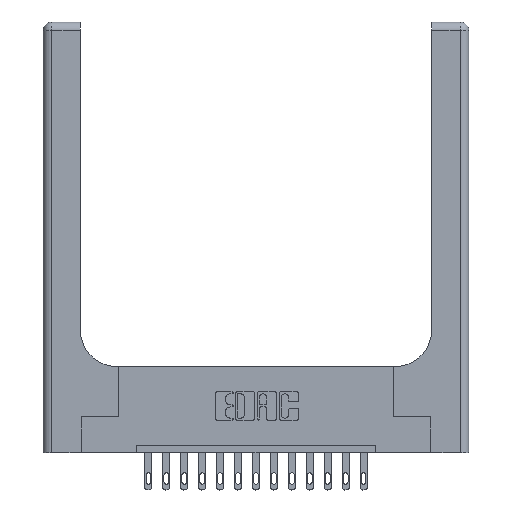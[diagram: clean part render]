
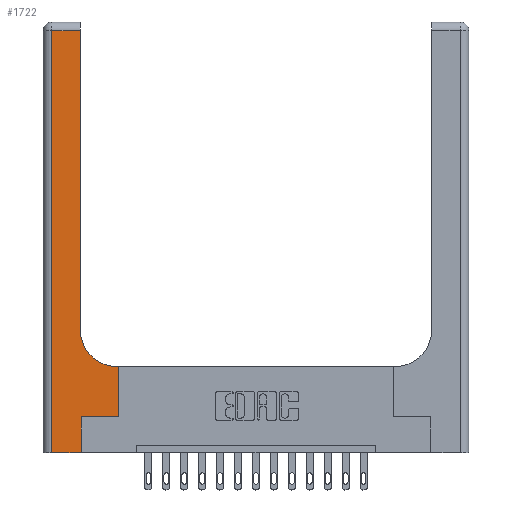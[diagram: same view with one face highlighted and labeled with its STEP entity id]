
A CAD part, top view. The second image highlights one B-rep face of the part: STEP entity #1722.
In plain terms, the highlighted planar face has unit normal (0, 0, 1).
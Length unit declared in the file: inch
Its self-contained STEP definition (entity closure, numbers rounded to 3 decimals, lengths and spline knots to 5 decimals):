
#23 = LINE ( 'NONE', #4002, #12143 ) ;
#140 = VERTEX_POINT ( 'NONE', #5116 ) ;
#315 = DIRECTION ( 'NONE',  ( 1., 0., 0. ) ) ;
#330 = VERTEX_POINT ( 'NONE', #6888 ) ;
#410 = EDGE_LOOP ( 'NONE', ( #9608, #13199, #13358, #5320, #7564, #8364, #5635, #8838, #11542 ) ) ;
#685 = CARTESIAN_POINT ( 'NONE',  ( 0., 0., 0.37 ) ) ;
#811 = LINE ( 'NONE', #2045, #11578 ) ;
#825 = CARTESIAN_POINT ( 'NONE',  ( 0.265, 0.25, 0.37 ) ) ;
#1722 = ADVANCED_FACE ( 'NONE', ( #9161 ), #14543, .F. ) ;
#2045 = CARTESIAN_POINT ( 'NONE',  ( 0.26, 0.6, 0.37 ) ) ;
#2172 = VECTOR ( 'NONE', #9384, 39.37008 ) ;
#2356 = AXIS2_PLACEMENT_3D ( 'NONE', #7818, #13225, #3804 ) ;
#2759 = AXIS2_PLACEMENT_3D ( 'NONE', #15444, #12954, #3292 ) ;
#3011 = LINE ( 'NONE', #3109, #15241 ) ;
#3109 = CARTESIAN_POINT ( 'NONE',  ( 0.06, 3., 0.37 ) ) ;
#3292 = DIRECTION ( 'NONE',  ( 1., 0., 0. ) ) ;
#3332 = VERTEX_POINT ( 'NONE', #16554 ) ;
#3633 = DIRECTION ( 'NONE',  ( 0., 1., 0. ) ) ;
#3804 = DIRECTION ( 'NONE',  ( -1., 0., 0. ) ) ;
#4002 = CARTESIAN_POINT ( 'NONE',  ( 0.528, 0.25, 0.37 ) ) ;
#4422 = DIRECTION ( 'NONE',  ( 0., -1., 0. ) ) ;
#5116 = CARTESIAN_POINT ( 'NONE',  ( 0.265, 0., 0.37 ) ) ;
#5320 = ORIENTED_EDGE ( 'NONE', *, *, #17372, .T. ) ;
#5635 = ORIENTED_EDGE ( 'NONE', *, *, #14506, .T. ) ;
#6217 = VECTOR ( 'NONE', #8687, 39.37008 ) ;
#6888 = CARTESIAN_POINT ( 'NONE',  ( 0.26, 0.85, 0.37 ) ) ;
#6954 = VERTEX_POINT ( 'NONE', #7953 ) ;
#7021 = EDGE_CURVE ( 'NONE', #14802, #6954, #8585, .T. ) ;
#7530 = CARTESIAN_POINT ( 'NONE',  ( 0.51, 0.6, 0.37 ) ) ;
#7564 = ORIENTED_EDGE ( 'NONE', *, *, #15340, .T. ) ;
#7727 = VECTOR ( 'NONE', #315, 39.37008 ) ;
#7818 = CARTESIAN_POINT ( 'NONE',  ( 0., 3., 0.37 ) ) ;
#7953 = CARTESIAN_POINT ( 'NONE',  ( 0.528, 0.25, 0.37 ) ) ;
#8364 = ORIENTED_EDGE ( 'NONE', *, *, #7021, .T. ) ;
#8383 = DIRECTION ( 'NONE',  ( 0., 1., 0. ) ) ;
#8492 = CARTESIAN_POINT ( 'NONE',  ( 0.265, 0.25, 0.37 ) ) ;
#8503 = CARTESIAN_POINT ( 'NONE',  ( 0.06, 0., 0.37 ) ) ;
#8585 = LINE ( 'NONE', #8492, #7727 ) ;
#8687 = DIRECTION ( 'NONE',  ( 1., 0., 0. ) ) ;
#8838 = ORIENTED_EDGE ( 'NONE', *, *, #15443, .T. ) ;
#9161 = FACE_OUTER_BOUND ( 'NONE', #410, .T. ) ;
#9234 = DIRECTION ( 'NONE',  ( 0., 1., 0. ) ) ;
#9318 = CARTESIAN_POINT ( 'NONE',  ( 0.26, 3., 0.37 ) ) ;
#9384 = DIRECTION ( 'NONE',  ( -1., 0., 0. ) ) ;
#9591 = VERTEX_POINT ( 'NONE', #12235 ) ;
#9608 = ORIENTED_EDGE ( 'NONE', *, *, #15599, .T. ) ;
#10144 = CIRCLE ( 'NONE', #2759, 0.25 ) ;
#10432 = VECTOR ( 'NONE', #3633, 39.37008 ) ;
#10658 = LINE ( 'NONE', #9318, #13247 ) ;
#11388 = VERTEX_POINT ( 'NONE', #8503 ) ;
#11542 = ORIENTED_EDGE ( 'NONE', *, *, #15437, .T. ) ;
#11578 = VECTOR ( 'NONE', #14455, 39.37008 ) ;
#12143 = VECTOR ( 'NONE', #8383, 39.37008 ) ;
#12235 = CARTESIAN_POINT ( 'NONE',  ( 0.528, 0.6, 0.37 ) ) ;
#12584 = EDGE_CURVE ( 'NONE', #16290, #3332, #15626, .T. ) ;
#12954 = DIRECTION ( 'NONE',  ( 0., 0., -1. ) ) ;
#13199 = ORIENTED_EDGE ( 'NONE', *, *, #12584, .T. ) ;
#13225 = DIRECTION ( 'NONE',  ( 0., 0., -1. ) ) ;
#13247 = VECTOR ( 'NONE', #9234, 39.37008 ) ;
#13358 = ORIENTED_EDGE ( 'NONE', *, *, #13958, .T. ) ;
#13958 = EDGE_CURVE ( 'NONE', #3332, #11388, #3011, .T. ) ;
#13985 = CARTESIAN_POINT ( 'NONE',  ( 0.26, 2.94, 0.37 ) ) ;
#14455 = DIRECTION ( 'NONE',  ( -1., 0., 0. ) ) ;
#14506 = EDGE_CURVE ( 'NONE', #6954, #9591, #23, .T. ) ;
#14543 = PLANE ( 'NONE',  #2356 ) ;
#14802 = VERTEX_POINT ( 'NONE', #825 ) ;
#15241 = VECTOR ( 'NONE', #4422, 39.37008 ) ;
#15340 = EDGE_CURVE ( 'NONE', #140, #14802, #15616, .T. ) ;
#15404 = LINE ( 'NONE', #685, #6217 ) ;
#15437 = EDGE_CURVE ( 'NONE', #17035, #330, #10144, .T. ) ;
#15443 = EDGE_CURVE ( 'NONE', #9591, #17035, #811, .T. ) ;
#15444 = CARTESIAN_POINT ( 'NONE',  ( 0.51, 0.85, 0.37 ) ) ;
#15599 = EDGE_CURVE ( 'NONE', #330, #16290, #10658, .T. ) ;
#15616 = LINE ( 'NONE', #16763, #10432 ) ;
#15626 = LINE ( 'NONE', #16945, #2172 ) ;
#16290 = VERTEX_POINT ( 'NONE', #13985 ) ;
#16554 = CARTESIAN_POINT ( 'NONE',  ( 0.06, 2.94, 0.37 ) ) ;
#16763 = CARTESIAN_POINT ( 'NONE',  ( 0.265, 0., 0.37 ) ) ;
#16945 = CARTESIAN_POINT ( 'NONE',  ( 0., 2.94, 0.37 ) ) ;
#17035 = VERTEX_POINT ( 'NONE', #7530 ) ;
#17372 = EDGE_CURVE ( 'NONE', #11388, #140, #15404, .T. ) ;
